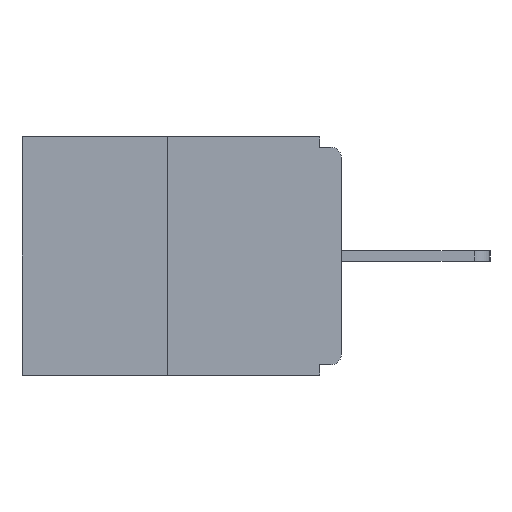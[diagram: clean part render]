
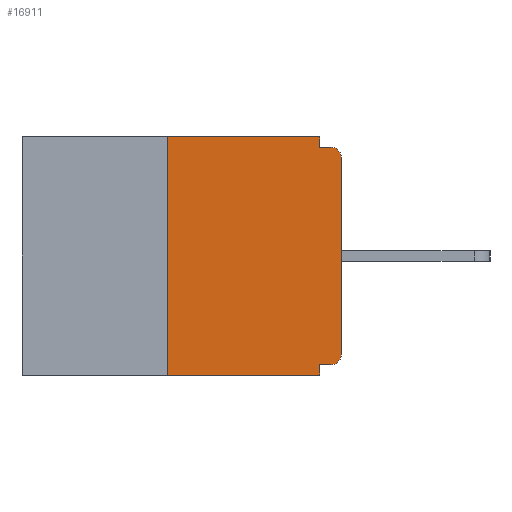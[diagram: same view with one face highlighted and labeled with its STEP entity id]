
A CAD part, left-side view. The second image highlights one B-rep face of the part: STEP entity #16911.
In plain terms, the highlighted planar face has unit normal (-1, 0, 0).
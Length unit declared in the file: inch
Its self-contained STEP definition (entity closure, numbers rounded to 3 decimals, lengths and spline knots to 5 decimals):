
#204 = CARTESIAN_POINT ( 'NONE',  ( 0., 0.015, -0.015 ) ) ;
#567 = DIRECTION ( 'NONE',  ( 0., 0., 1. ) ) ;
#631 = ORIENTED_EDGE ( 'NONE', *, *, #13217, .T. ) ;
#653 = VECTOR ( 'NONE', #18437, 39.37008 ) ;
#705 = DIRECTION ( 'NONE',  ( 0., 0., 1. ) ) ;
#997 = EDGE_LOOP ( 'NONE', ( #18004, #6620, #2475, #6339, #7934, #7047, #18459, #631, #6652, #14351 ) ) ;
#1204 = DIRECTION ( 'NONE',  ( 0., -1., 0. ) ) ;
#1672 = EDGE_CURVE ( 'NONE', #21219, #17258, #17878, .T. ) ;
#2475 = ORIENTED_EDGE ( 'NONE', *, *, #22608, .T. ) ;
#2542 = EDGE_CURVE ( 'NONE', #5494, #13866, #6442, .T. ) ;
#2854 = CARTESIAN_POINT ( 'NONE',  ( 0., 0.46, 0. ) ) ;
#3424 = CARTESIAN_POINT ( 'NONE',  ( 0., 0.25, -0.343 ) ) ;
#3708 = VECTOR ( 'NONE', #567, 39.37008 ) ;
#3998 = LINE ( 'NONE', #9726, #11437 ) ;
#4356 = CARTESIAN_POINT ( 'NONE',  ( 0., 0., 0. ) ) ;
#4400 = DIRECTION ( 'NONE',  ( 0., -1., 0. ) ) ;
#4528 = EDGE_CURVE ( 'NONE', #17258, #14532, #16969, .T. ) ;
#4632 = VECTOR ( 'NONE', #1204, 39.37008 ) ;
#4698 = DIRECTION ( 'NONE',  ( 0., 1., 0. ) ) ;
#4728 = CARTESIAN_POINT ( 'NONE',  ( 0., 0., -0.03 ) ) ;
#4898 = VECTOR ( 'NONE', #705, 39.37008 ) ;
#4997 = DIRECTION ( 'NONE',  ( 0., 0., -1. ) ) ;
#5494 = VERTEX_POINT ( 'NONE', #12356 ) ;
#5924 = CARTESIAN_POINT ( 'NONE',  ( 0., 0., -0.313 ) ) ;
#6120 = VECTOR ( 'NONE', #4698, 39.37008 ) ;
#6207 = CARTESIAN_POINT ( 'NONE',  ( 0., 0.031, -0.343 ) ) ;
#6339 = ORIENTED_EDGE ( 'NONE', *, *, #2542, .F. ) ;
#6442 = LINE ( 'NONE', #11793, #14869 ) ;
#6609 = EDGE_CURVE ( 'NONE', #21219, #5494, #8276, .T. ) ;
#6620 = ORIENTED_EDGE ( 'NONE', *, *, #16827, .F. ) ;
#6652 = ORIENTED_EDGE ( 'NONE', *, *, #15052, .F. ) ;
#7047 = ORIENTED_EDGE ( 'NONE', *, *, #1672, .T. ) ;
#7417 = LINE ( 'NONE', #14413, #653 ) ;
#7688 = VECTOR ( 'NONE', #4400, 39.37008 ) ;
#7934 = ORIENTED_EDGE ( 'NONE', *, *, #6609, .F. ) ;
#8102 = PLANE ( 'NONE',  #9867 ) ;
#8212 = LINE ( 'NONE', #16999, #4898 ) ;
#8232 = LINE ( 'NONE', #15249, #7688 ) ;
#8276 = LINE ( 'NONE', #13749, #6120 ) ;
#9726 = CARTESIAN_POINT ( 'NONE',  ( 0., 0.031, 0. ) ) ;
#9867 = AXIS2_PLACEMENT_3D ( 'NONE', #2854, #15341, #11773 ) ;
#9965 = AXIS2_PLACEMENT_3D ( 'NONE', #14196, #13357, #16696 ) ;
#10136 = LINE ( 'NONE', #15463, #4632 ) ;
#11437 = VECTOR ( 'NONE', #20163, 39.37008 ) ;
#11773 = DIRECTION ( 'NONE',  ( 0., 0., -1. ) ) ;
#11793 = CARTESIAN_POINT ( 'NONE',  ( 0., 0.031, -0.343 ) ) ;
#12356 = CARTESIAN_POINT ( 'NONE',  ( 0., 0.031, -0.328 ) ) ;
#12362 = DIRECTION ( 'NONE',  ( -1., 0., 0. ) ) ;
#12866 = VERTEX_POINT ( 'NONE', #20612 ) ;
#13217 = EDGE_CURVE ( 'NONE', #14532, #15927, #14116, .T. ) ;
#13357 = DIRECTION ( 'NONE',  ( -1., 0., 0. ) ) ;
#13749 = CARTESIAN_POINT ( 'NONE',  ( 0., 0., -0.328 ) ) ;
#13866 = VERTEX_POINT ( 'NONE', #6207 ) ;
#13896 = CARTESIAN_POINT ( 'NONE',  ( 0., 0.015, -0.313 ) ) ;
#13930 = CARTESIAN_POINT ( 'NONE',  ( 0., 0.031, 0. ) ) ;
#14116 = CIRCLE ( 'NONE', #9965, 0.015 ) ;
#14196 = CARTESIAN_POINT ( 'NONE',  ( 0., 0.015, -0.03 ) ) ;
#14351 = ORIENTED_EDGE ( 'NONE', *, *, #21076, .F. ) ;
#14413 = CARTESIAN_POINT ( 'NONE',  ( 0., 0., -0.015 ) ) ;
#14532 = VERTEX_POINT ( 'NONE', #4728 ) ;
#14869 = VECTOR ( 'NONE', #4997, 39.37008 ) ;
#15052 = EDGE_CURVE ( 'NONE', #12866, #15927, #7417, .T. ) ;
#15249 = CARTESIAN_POINT ( 'NONE',  ( 0., 0.46, -0.343 ) ) ;
#15341 = DIRECTION ( 'NONE',  ( 1., 0., 0. ) ) ;
#15463 = CARTESIAN_POINT ( 'NONE',  ( 0., 0.46, 0. ) ) ;
#15927 = VERTEX_POINT ( 'NONE', #204 ) ;
#16549 = VERTEX_POINT ( 'NONE', #20604 ) ;
#16696 = DIRECTION ( 'NONE',  ( 0., 0., -1. ) ) ;
#16827 = EDGE_CURVE ( 'NONE', #20999, #16549, #8212, .T. ) ;
#16911 = ADVANCED_FACE ( 'NONE', ( #20105 ), #8102, .F. ) ;
#16969 = LINE ( 'NONE', #4356, #3708 ) ;
#16999 = CARTESIAN_POINT ( 'NONE',  ( 0., 0.25, 0. ) ) ;
#17258 = VERTEX_POINT ( 'NONE', #5924 ) ;
#17878 = CIRCLE ( 'NONE', #20905, 0.015 ) ;
#18004 = ORIENTED_EDGE ( 'NONE', *, *, #22590, .F. ) ;
#18437 = DIRECTION ( 'NONE',  ( 0., -1., 0. ) ) ;
#18459 = ORIENTED_EDGE ( 'NONE', *, *, #4528, .T. ) ;
#19359 = DIRECTION ( 'NONE',  ( 0., 0., -1. ) ) ;
#20105 = FACE_OUTER_BOUND ( 'NONE', #997, .T. ) ;
#20163 = DIRECTION ( 'NONE',  ( 0., 0., -1. ) ) ;
#20604 = CARTESIAN_POINT ( 'NONE',  ( 0., 0.25, 0. ) ) ;
#20612 = CARTESIAN_POINT ( 'NONE',  ( 0., 0.031, -0.015 ) ) ;
#20905 = AXIS2_PLACEMENT_3D ( 'NONE', #13896, #12362, #19359 ) ;
#20982 = CARTESIAN_POINT ( 'NONE',  ( 0., 0.015, -0.328 ) ) ;
#20999 = VERTEX_POINT ( 'NONE', #3424 ) ;
#21076 = EDGE_CURVE ( 'NONE', #22145, #12866, #3998, .T. ) ;
#21219 = VERTEX_POINT ( 'NONE', #20982 ) ;
#22145 = VERTEX_POINT ( 'NONE', #13930 ) ;
#22590 = EDGE_CURVE ( 'NONE', #16549, #22145, #10136, .T. ) ;
#22608 = EDGE_CURVE ( 'NONE', #20999, #13866, #8232, .T. ) ;
